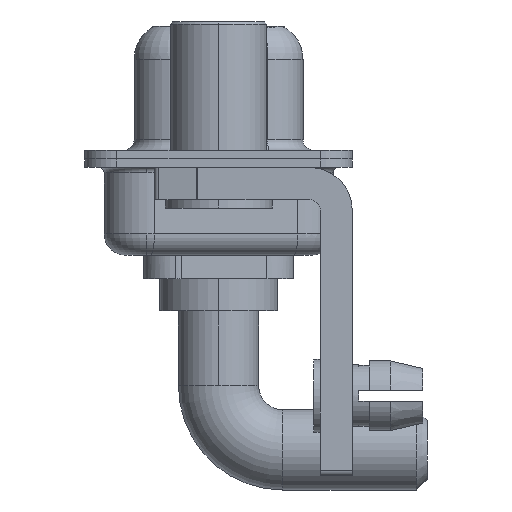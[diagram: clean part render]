
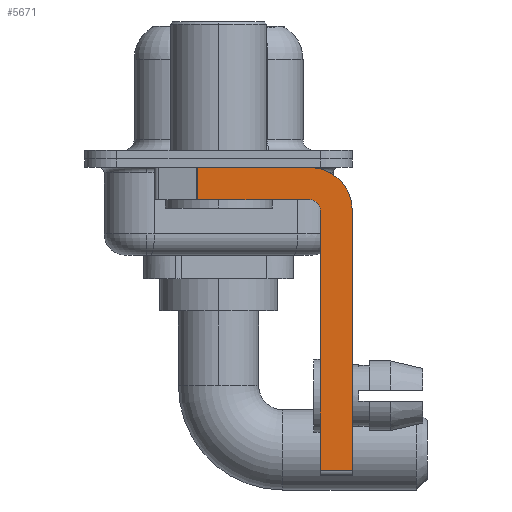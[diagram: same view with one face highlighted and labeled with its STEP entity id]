
A CAD part, left-side view. The second image highlights one B-rep face of the part: STEP entity #5671.
In plain terms, the highlighted planar face has unit normal (-1, 0, 0).
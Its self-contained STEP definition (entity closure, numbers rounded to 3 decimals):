
#50 = CARTESIAN_POINT ( 'NONE',  ( -2.9, -4.25, -2.4 ) ) ;
#504 = VERTEX_POINT ( 'NONE', #6822 ) ;
#689 = EDGE_CURVE ( 'NONE', #8453, #1781, #9903, .T. ) ;
#930 = VERTEX_POINT ( 'NONE', #2219 ) ;
#1022 = DIRECTION ( 'NONE',  ( 0., 0., -1. ) ) ;
#1192 = ORIENTED_EDGE ( 'NONE', *, *, #4598, .F. ) ;
#1259 = FACE_OUTER_BOUND ( 'NONE', #2687, .T. ) ;
#1420 = CARTESIAN_POINT ( 'NONE',  ( -2.9, 3., -0.4 ) ) ;
#1595 = DIRECTION ( 'NONE',  ( 0., -1., 0. ) ) ;
#1621 = DIRECTION ( 'NONE',  ( 0., -1., 0. ) ) ;
#1781 = VERTEX_POINT ( 'NONE', #4127 ) ;
#1992 = AXIS2_PLACEMENT_3D ( 'NONE', #50, #11997, #8311 ) ;
#2219 = CARTESIAN_POINT ( 'NONE',  ( -2.9, -4.75, -2.4 ) ) ;
#2411 = LINE ( 'NONE', #11920, #10348 ) ;
#2459 = DIRECTION ( 'NONE',  ( 0., 0., -1. ) ) ;
#2656 = EDGE_CURVE ( 'NONE', #15494, #1781, #2411, .T. ) ;
#2687 = EDGE_LOOP ( 'NONE', ( #14389, #16670, #9939, #3314, #1192, #6985, #9889, #6037 ) ) ;
#3170 = CARTESIAN_POINT ( 'NONE',  ( -2.9, -6.25, -2.4 ) ) ;
#3192 = CARTESIAN_POINT ( 'NONE',  ( -2.9, -4.25, -14.55 ) ) ;
#3314 = ORIENTED_EDGE ( 'NONE', *, *, #15156, .F. ) ;
#3318 = AXIS2_PLACEMENT_3D ( 'NONE', #7571, #9158, #2459 ) ;
#4127 = CARTESIAN_POINT ( 'NONE',  ( -2.9, -6.25, -14.55 ) ) ;
#4598 = EDGE_CURVE ( 'NONE', #8453, #930, #13715, .T. ) ;
#4727 = VERTEX_POINT ( 'NONE', #9752 ) ;
#4753 = VECTOR ( 'NONE', #1621, 1000. ) ;
#5043 = VERTEX_POINT ( 'NONE', #17417 ) ;
#5671 = ADVANCED_FACE ( 'NONE', ( #1259 ), #8222, .F. ) ;
#6023 = EDGE_CURVE ( 'NONE', #5043, #504, #15795, .T. ) ;
#6037 = ORIENTED_EDGE ( 'NONE', *, *, #15772, .F. ) ;
#6822 = CARTESIAN_POINT ( 'NONE',  ( -2.9, 0.978, -1.9 ) ) ;
#6985 = ORIENTED_EDGE ( 'NONE', *, *, #689, .T. ) ;
#7559 = CIRCLE ( 'NONE', #3318, 2. ) ;
#7571 = CARTESIAN_POINT ( 'NONE',  ( -2.9, -4.25, -2.4 ) ) ;
#7607 = VECTOR ( 'NONE', #8910, 1000. ) ;
#8078 = DIRECTION ( 'NONE',  ( 0., 0., 1. ) ) ;
#8222 = PLANE ( 'NONE',  #1992 ) ;
#8311 = DIRECTION ( 'NONE',  ( 0., 0., -1. ) ) ;
#8453 = VERTEX_POINT ( 'NONE', #15482 ) ;
#8910 = DIRECTION ( 'NONE',  ( 0., 1., 0. ) ) ;
#8947 = AXIS2_PLACEMENT_3D ( 'NONE', #10164, #15543, #17318 ) ;
#9158 = DIRECTION ( 'NONE',  ( 1., 0., 0. ) ) ;
#9752 = CARTESIAN_POINT ( 'NONE',  ( -2.9, -4.25, -0.4 ) ) ;
#9889 = ORIENTED_EDGE ( 'NONE', *, *, #2656, .F. ) ;
#9903 = LINE ( 'NONE', #3192, #4753 ) ;
#9939 = ORIENTED_EDGE ( 'NONE', *, *, #6023, .F. ) ;
#10164 = CARTESIAN_POINT ( 'NONE',  ( -2.9, -4.25, -2.4 ) ) ;
#10348 = VECTOR ( 'NONE', #11835, 1000. ) ;
#10367 = LINE ( 'NONE', #11592, #17002 ) ;
#10526 = VECTOR ( 'NONE', #1595, 1000. ) ;
#11278 = EDGE_CURVE ( 'NONE', #17278, #504, #10367, .T. ) ;
#11505 = VECTOR ( 'NONE', #8078, 1000. ) ;
#11592 = CARTESIAN_POINT ( 'NONE',  ( -2.9, 0.978, -1.9 ) ) ;
#11717 = CARTESIAN_POINT ( 'NONE',  ( -2.9, -4.25, -1.9 ) ) ;
#11835 = DIRECTION ( 'NONE',  ( 0., 0., -1. ) ) ;
#11920 = CARTESIAN_POINT ( 'NONE',  ( -2.9, -6.25, -2.4 ) ) ;
#11997 = DIRECTION ( 'NONE',  ( 1., 0., 0. ) ) ;
#12283 = EDGE_CURVE ( 'NONE', #17278, #4727, #15010, .T. ) ;
#13715 = LINE ( 'NONE', #16021, #11505 ) ;
#14288 = CIRCLE ( 'NONE', #8947, 0.5 ) ;
#14389 = ORIENTED_EDGE ( 'NONE', *, *, #12283, .F. ) ;
#15010 = LINE ( 'NONE', #1420, #10526 ) ;
#15156 = EDGE_CURVE ( 'NONE', #930, #5043, #14288, .T. ) ;
#15482 = CARTESIAN_POINT ( 'NONE',  ( -2.9, -4.75, -14.55 ) ) ;
#15494 = VERTEX_POINT ( 'NONE', #3170 ) ;
#15543 = DIRECTION ( 'NONE',  ( -1., 0., 0. ) ) ;
#15772 = EDGE_CURVE ( 'NONE', #4727, #15494, #7559, .T. ) ;
#15795 = LINE ( 'NONE', #11717, #7607 ) ;
#16021 = CARTESIAN_POINT ( 'NONE',  ( -2.9, -4.75, -14.8 ) ) ;
#16392 = CARTESIAN_POINT ( 'NONE',  ( -2.9, 0.978, -0.4 ) ) ;
#16670 = ORIENTED_EDGE ( 'NONE', *, *, #11278, .T. ) ;
#17002 = VECTOR ( 'NONE', #1022, 1000. ) ;
#17278 = VERTEX_POINT ( 'NONE', #16392 ) ;
#17318 = DIRECTION ( 'NONE',  ( 0., 0., 1. ) ) ;
#17417 = CARTESIAN_POINT ( 'NONE',  ( -2.9, -4.25, -1.9 ) ) ;
